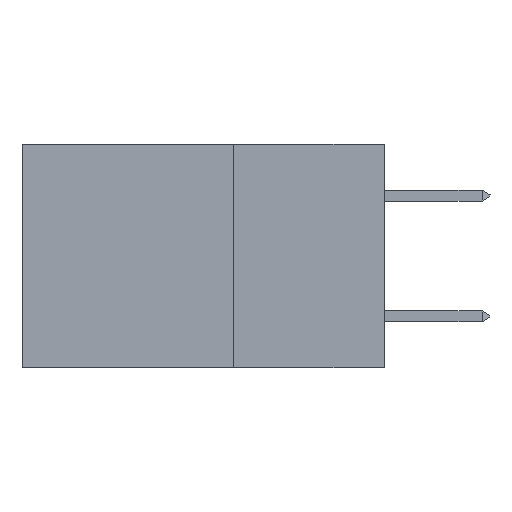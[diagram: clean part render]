
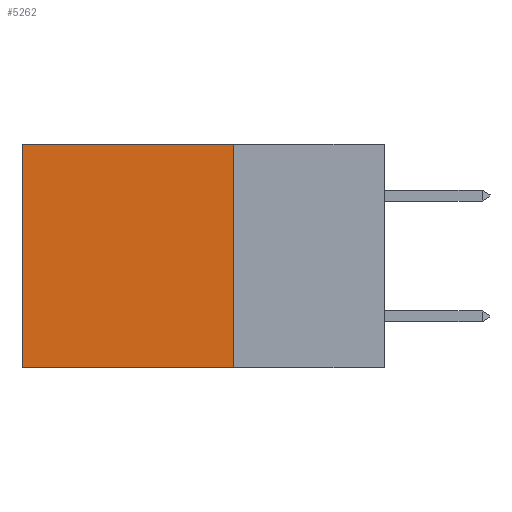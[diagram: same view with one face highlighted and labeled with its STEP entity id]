
A CAD part, left-side view. The second image highlights one B-rep face of the part: STEP entity #5262.
In plain terms, the highlighted planar face has unit normal (-1, 0, 0).
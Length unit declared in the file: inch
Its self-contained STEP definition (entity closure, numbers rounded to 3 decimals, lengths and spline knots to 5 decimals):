
#214 = CARTESIAN_POINT ( 'NONE',  ( 0.2875, 0.25, 0. ) ) ;
#267 = LINE ( 'NONE', #486, #4632 ) ;
#486 = CARTESIAN_POINT ( 'NONE',  ( 0.2875, 0.25, -0.37 ) ) ;
#982 = VECTOR ( 'NONE', #12118, 39.37008 ) ;
#1736 = DIRECTION ( 'NONE',  ( 0., 0., -1. ) ) ;
#1750 = CARTESIAN_POINT ( 'NONE',  ( 0.2875, 0.6, -0.37 ) ) ;
#2165 = CARTESIAN_POINT ( 'NONE',  ( 0.2875, 0.6, 0. ) ) ;
#2521 = EDGE_CURVE ( 'NONE', #7489, #9785, #18942, .T. ) ;
#2618 = CARTESIAN_POINT ( 'NONE',  ( 0.2875, 0.25, 0. ) ) ;
#3104 = DIRECTION ( 'NONE',  ( 1., 0., 0. ) ) ;
#3319 = ORIENTED_EDGE ( 'NONE', *, *, #2521, .T. ) ;
#3513 = CARTESIAN_POINT ( 'NONE',  ( 0.2875, 0.6, 0. ) ) ;
#4632 = VECTOR ( 'NONE', #18245, 39.37008 ) ;
#5262 = ADVANCED_FACE ( 'NONE', ( #11246 ), #19681, .F. ) ;
#5579 = CARTESIAN_POINT ( 'NONE',  ( 0.2875, 0.25, 0. ) ) ;
#5933 = DIRECTION ( 'NONE',  ( 0., 0., -1. ) ) ;
#7489 = VERTEX_POINT ( 'NONE', #2618 ) ;
#9366 = LINE ( 'NONE', #19199, #11958 ) ;
#9785 = VERTEX_POINT ( 'NONE', #3513 ) ;
#10670 = VECTOR ( 'NONE', #1736, 39.37008 ) ;
#11246 = FACE_OUTER_BOUND ( 'NONE', #19836, .T. ) ;
#11958 = VECTOR ( 'NONE', #5933, 39.37008 ) ;
#12118 = DIRECTION ( 'NONE',  ( 0., 1., 0. ) ) ;
#12562 = ORIENTED_EDGE ( 'NONE', *, *, #21103, .T. ) ;
#13258 = VERTEX_POINT ( 'NONE', #15897 ) ;
#13614 = EDGE_CURVE ( 'NONE', #13258, #13853, #267, .T. ) ;
#13853 = VERTEX_POINT ( 'NONE', #1750 ) ;
#14723 = ORIENTED_EDGE ( 'NONE', *, *, #13614, .F. ) ;
#15897 = CARTESIAN_POINT ( 'NONE',  ( 0.2875, 0.25, -0.37 ) ) ;
#16497 = LINE ( 'NONE', #2165, #10670 ) ;
#17706 = ORIENTED_EDGE ( 'NONE', *, *, #19386, .F. ) ;
#18083 = AXIS2_PLACEMENT_3D ( 'NONE', #214, #3104, #19367 ) ;
#18245 = DIRECTION ( 'NONE',  ( 0., 1., 0. ) ) ;
#18942 = LINE ( 'NONE', #5579, #982 ) ;
#19199 = CARTESIAN_POINT ( 'NONE',  ( 0.2875, 0.25, 0. ) ) ;
#19367 = DIRECTION ( 'NONE',  ( 0., 0., -1. ) ) ;
#19386 = EDGE_CURVE ( 'NONE', #7489, #13258, #9366, .T. ) ;
#19681 = PLANE ( 'NONE',  #18083 ) ;
#19836 = EDGE_LOOP ( 'NONE', ( #12562, #14723, #17706, #3319 ) ) ;
#21103 = EDGE_CURVE ( 'NONE', #9785, #13853, #16497, .T. ) ;
